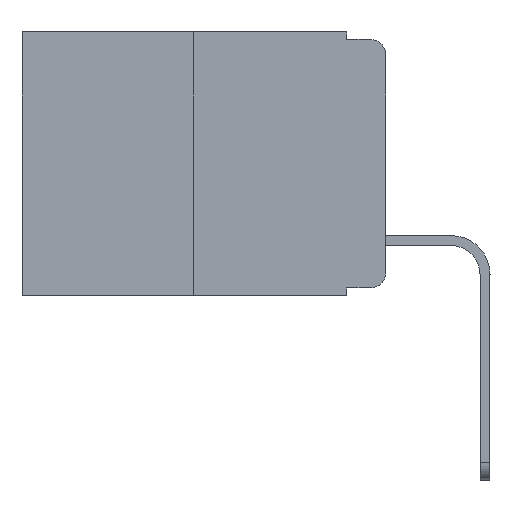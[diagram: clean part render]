
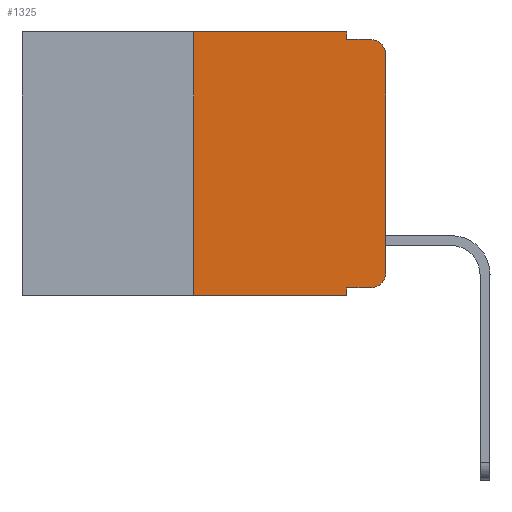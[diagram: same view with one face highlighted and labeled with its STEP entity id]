
A CAD part, left-side view. The second image highlights one B-rep face of the part: STEP entity #1325.
In plain terms, the highlighted planar face has unit normal (-1, 0, 0).
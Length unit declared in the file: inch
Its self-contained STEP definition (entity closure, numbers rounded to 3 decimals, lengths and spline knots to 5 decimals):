
#82 = DIRECTION ( 'NONE',  ( 0., 0., -1. ) ) ;
#227 = VECTOR ( 'NONE', #7457, 39.37008 ) ;
#311 = CARTESIAN_POINT ( 'NONE',  ( 0., 0.473, -0.343 ) ) ;
#336 = DIRECTION ( 'NONE',  ( 0., 0., -1. ) ) ;
#396 = CARTESIAN_POINT ( 'NONE',  ( 0., 0.051, -0.333 ) ) ;
#543 = VECTOR ( 'NONE', #3770, 39.37008 ) ;
#714 = ORIENTED_EDGE ( 'NONE', *, *, #1074, .F. ) ;
#995 = VERTEX_POINT ( 'NONE', #3834 ) ;
#1069 = ORIENTED_EDGE ( 'NONE', *, *, #1538, .F. ) ;
#1074 = EDGE_CURVE ( 'NONE', #5106, #6589, #3025, .T. ) ;
#1225 = CIRCLE ( 'NONE', #9360, 0.02 ) ;
#1325 = ADVANCED_FACE ( 'NONE', ( #6968 ), #3450, .F. ) ;
#1505 = DIRECTION ( 'NONE',  ( -1., 0., 0. ) ) ;
#1538 = EDGE_CURVE ( 'NONE', #8156, #6734, #2199, .T. ) ;
#1700 = LINE ( 'NONE', #8389, #543 ) ;
#1907 = DIRECTION ( 'NONE',  ( 0., -1., 0. ) ) ;
#2127 = ORIENTED_EDGE ( 'NONE', *, *, #5605, .F. ) ;
#2199 = LINE ( 'NONE', #6025, #227 ) ;
#2299 = VERTEX_POINT ( 'NONE', #8691 ) ;
#2325 = ORIENTED_EDGE ( 'NONE', *, *, #3788, .T. ) ;
#2360 = CARTESIAN_POINT ( 'NONE',  ( 0., 0., 0. ) ) ;
#2633 = ORIENTED_EDGE ( 'NONE', *, *, #7127, .F. ) ;
#2678 = DIRECTION ( 'NONE',  ( 0., 0., -1. ) ) ;
#2718 = VECTOR ( 'NONE', #9065, 39.37008 ) ;
#3025 = LINE ( 'NONE', #4447, #8752 ) ;
#3057 = CARTESIAN_POINT ( 'NONE',  ( 0., 0.02, -0.313 ) ) ;
#3152 = ORIENTED_EDGE ( 'NONE', *, *, #4497, .T. ) ;
#3450 = PLANE ( 'NONE',  #8035 ) ;
#3508 = VERTEX_POINT ( 'NONE', #7176 ) ;
#3770 = DIRECTION ( 'NONE',  ( 0., -1., 0. ) ) ;
#3788 = EDGE_CURVE ( 'NONE', #2299, #6413, #8572, .T. ) ;
#3834 = CARTESIAN_POINT ( 'NONE',  ( 0., 0.02, -0.333 ) ) ;
#4190 = DIRECTION ( 'NONE',  ( 0., 0., -1. ) ) ;
#4260 = CARTESIAN_POINT ( 'NONE',  ( 0., 0.051, 0. ) ) ;
#4266 = CIRCLE ( 'NONE', #5206, 0.02 ) ;
#4447 = CARTESIAN_POINT ( 'NONE',  ( 0., 0.051, -0.01 ) ) ;
#4497 = EDGE_CURVE ( 'NONE', #8156, #9147, #5976, .T. ) ;
#4657 = DIRECTION ( 'NONE',  ( 0., -1., 0. ) ) ;
#4929 = DIRECTION ( 'NONE',  ( 1., 0., 0. ) ) ;
#5106 = VERTEX_POINT ( 'NONE', #8177 ) ;
#5206 = AXIS2_PLACEMENT_3D ( 'NONE', #3057, #5973, #82 ) ;
#5605 = EDGE_CURVE ( 'NONE', #3508, #5106, #8560, .T. ) ;
#5973 = DIRECTION ( 'NONE',  ( -1., 0., 0. ) ) ;
#5976 = LINE ( 'NONE', #311, #7521 ) ;
#5978 = ORIENTED_EDGE ( 'NONE', *, *, #8673, .F. ) ;
#6025 = CARTESIAN_POINT ( 'NONE',  ( 0., 0.25, 0. ) ) ;
#6141 = DIRECTION ( 'NONE',  ( 0., -1., 0. ) ) ;
#6143 = LINE ( 'NONE', #4260, #7565 ) ;
#6321 = CARTESIAN_POINT ( 'NONE',  ( 0., 0.473, 0. ) ) ;
#6369 = DIRECTION ( 'NONE',  ( 0., 0., -1. ) ) ;
#6413 = VERTEX_POINT ( 'NONE', #7498 ) ;
#6540 = VECTOR ( 'NONE', #6369, 39.37008 ) ;
#6575 = CARTESIAN_POINT ( 'NONE',  ( 0., 0.02, -0.03 ) ) ;
#6589 = VERTEX_POINT ( 'NONE', #7742 ) ;
#6662 = CARTESIAN_POINT ( 'NONE',  ( 0., 0.25, 0. ) ) ;
#6691 = LINE ( 'NONE', #396, #7284 ) ;
#6734 = VERTEX_POINT ( 'NONE', #6662 ) ;
#6944 = ORIENTED_EDGE ( 'NONE', *, *, #9645, .T. ) ;
#6968 = FACE_OUTER_BOUND ( 'NONE', #8374, .T. ) ;
#7127 = EDGE_CURVE ( 'NONE', #9043, #9147, #6143, .T. ) ;
#7176 = CARTESIAN_POINT ( 'NONE',  ( 0., 0.051, 0. ) ) ;
#7240 = CARTESIAN_POINT ( 'NONE',  ( 0., 0.051, -0.333 ) ) ;
#7284 = VECTOR ( 'NONE', #1907, 39.37008 ) ;
#7457 = DIRECTION ( 'NONE',  ( 0., 0., 1. ) ) ;
#7488 = CARTESIAN_POINT ( 'NONE',  ( 0., 0.051, -0.343 ) ) ;
#7498 = CARTESIAN_POINT ( 'NONE',  ( 0., 0., -0.03 ) ) ;
#7521 = VECTOR ( 'NONE', #6141, 39.37008 ) ;
#7565 = VECTOR ( 'NONE', #2678, 39.37008 ) ;
#7742 = CARTESIAN_POINT ( 'NONE',  ( 0., 0.02, -0.01 ) ) ;
#7773 = ORIENTED_EDGE ( 'NONE', *, *, #8949, .T. ) ;
#7949 = ORIENTED_EDGE ( 'NONE', *, *, #8596, .T. ) ;
#8035 = AXIS2_PLACEMENT_3D ( 'NONE', #6321, #4929, #4190 ) ;
#8156 = VERTEX_POINT ( 'NONE', #9211 ) ;
#8177 = CARTESIAN_POINT ( 'NONE',  ( 0., 0.051, -0.01 ) ) ;
#8374 = EDGE_LOOP ( 'NONE', ( #2325, #6944, #714, #2127, #5978, #1069, #3152, #2633, #7773, #7949 ) ) ;
#8389 = CARTESIAN_POINT ( 'NONE',  ( 0., 0.473, 0. ) ) ;
#8560 = LINE ( 'NONE', #8681, #6540 ) ;
#8572 = LINE ( 'NONE', #2360, #2718 ) ;
#8596 = EDGE_CURVE ( 'NONE', #995, #2299, #4266, .T. ) ;
#8673 = EDGE_CURVE ( 'NONE', #6734, #3508, #1700, .T. ) ;
#8681 = CARTESIAN_POINT ( 'NONE',  ( 0., 0.051, 0. ) ) ;
#8691 = CARTESIAN_POINT ( 'NONE',  ( 0., 0., -0.313 ) ) ;
#8752 = VECTOR ( 'NONE', #4657, 39.37008 ) ;
#8949 = EDGE_CURVE ( 'NONE', #9043, #995, #6691, .T. ) ;
#9043 = VERTEX_POINT ( 'NONE', #7240 ) ;
#9065 = DIRECTION ( 'NONE',  ( 0., 0., 1. ) ) ;
#9147 = VERTEX_POINT ( 'NONE', #7488 ) ;
#9211 = CARTESIAN_POINT ( 'NONE',  ( 0., 0.25, -0.343 ) ) ;
#9360 = AXIS2_PLACEMENT_3D ( 'NONE', #6575, #1505, #336 ) ;
#9645 = EDGE_CURVE ( 'NONE', #6413, #6589, #1225, .T. ) ;
